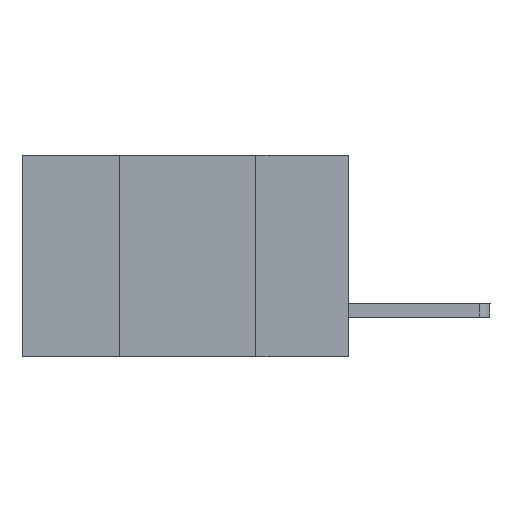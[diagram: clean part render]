
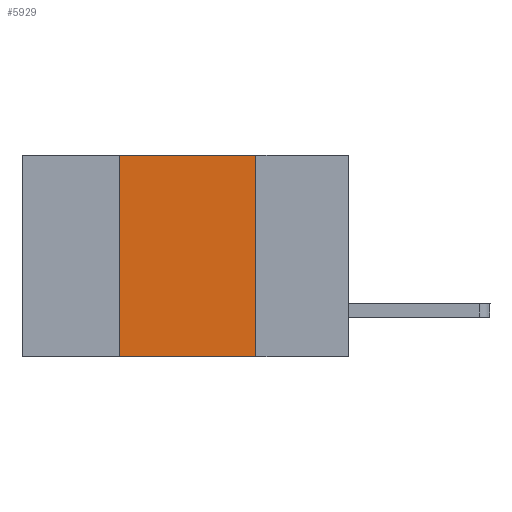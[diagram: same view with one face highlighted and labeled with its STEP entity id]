
A CAD part, left-side view. The second image highlights one B-rep face of the part: STEP entity #5929.
In plain terms, the highlighted planar face has unit normal (-1, 0, 0).
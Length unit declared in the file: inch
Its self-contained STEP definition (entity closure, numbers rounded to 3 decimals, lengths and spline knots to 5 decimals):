
#248 = CARTESIAN_POINT ( 'NONE',  ( 0., 0.17, -0.37 ) ) ;
#290 = LINE ( 'NONE', #248, #4316 ) ;
#458 = VERTEX_POINT ( 'NONE', #3441 ) ;
#1166 = ORIENTED_EDGE ( 'NONE', *, *, #3712, .F. ) ;
#1668 = PLANE ( 'NONE',  #8245 ) ;
#1730 = ORIENTED_EDGE ( 'NONE', *, *, #8825, .F. ) ;
#1849 = CARTESIAN_POINT ( 'NONE',  ( 0., 0.42, -0.37 ) ) ;
#2071 = VECTOR ( 'NONE', #8659, 39.37008 ) ;
#2373 = ORIENTED_EDGE ( 'NONE', *, *, #7870, .F. ) ;
#2729 = LINE ( 'NONE', #5010, #2071 ) ;
#2766 = CARTESIAN_POINT ( 'NONE',  ( 0., 0.6, -0.37 ) ) ;
#2989 = CARTESIAN_POINT ( 'NONE',  ( 0., 0.42, -0.37 ) ) ;
#3441 = CARTESIAN_POINT ( 'NONE',  ( 0., 0.17, -0.37 ) ) ;
#3712 = EDGE_CURVE ( 'NONE', #5373, #458, #290, .T. ) ;
#3832 = VERTEX_POINT ( 'NONE', #6043 ) ;
#4238 = VERTEX_POINT ( 'NONE', #2989 ) ;
#4316 = VECTOR ( 'NONE', #5694, 39.37008 ) ;
#4380 = VECTOR ( 'NONE', #7763, 39.37008 ) ;
#4436 = CARTESIAN_POINT ( 'NONE',  ( 0., 0.6, 0. ) ) ;
#4578 = DIRECTION ( 'NONE',  ( 1., 0., 0. ) ) ;
#4832 = EDGE_CURVE ( 'NONE', #4238, #458, #7964, .T. ) ;
#5010 = CARTESIAN_POINT ( 'NONE',  ( 0., 0.6, 0. ) ) ;
#5373 = VERTEX_POINT ( 'NONE', #9369 ) ;
#5694 = DIRECTION ( 'NONE',  ( 0., 0., -1. ) ) ;
#5929 = ADVANCED_FACE ( 'NONE', ( #8271 ), #1668, .F. ) ;
#6043 = CARTESIAN_POINT ( 'NONE',  ( 0., 0.42, 0. ) ) ;
#6986 = VECTOR ( 'NONE', #8690, 39.37008 ) ;
#7281 = ORIENTED_EDGE ( 'NONE', *, *, #4832, .T. ) ;
#7763 = DIRECTION ( 'NONE',  ( 0., 0., 1. ) ) ;
#7870 = EDGE_CURVE ( 'NONE', #4238, #3832, #8502, .T. ) ;
#7964 = LINE ( 'NONE', #2766, #6986 ) ;
#8175 = DIRECTION ( 'NONE',  ( 0., 0., -1. ) ) ;
#8245 = AXIS2_PLACEMENT_3D ( 'NONE', #4436, #4578, #8175 ) ;
#8271 = FACE_OUTER_BOUND ( 'NONE', #9191, .T. ) ;
#8502 = LINE ( 'NONE', #1849, #4380 ) ;
#8659 = DIRECTION ( 'NONE',  ( 0., -1., 0. ) ) ;
#8690 = DIRECTION ( 'NONE',  ( 0., -1., 0. ) ) ;
#8825 = EDGE_CURVE ( 'NONE', #3832, #5373, #2729, .T. ) ;
#9191 = EDGE_LOOP ( 'NONE', ( #1166, #1730, #2373, #7281 ) ) ;
#9369 = CARTESIAN_POINT ( 'NONE',  ( 0., 0.17, 0. ) ) ;
